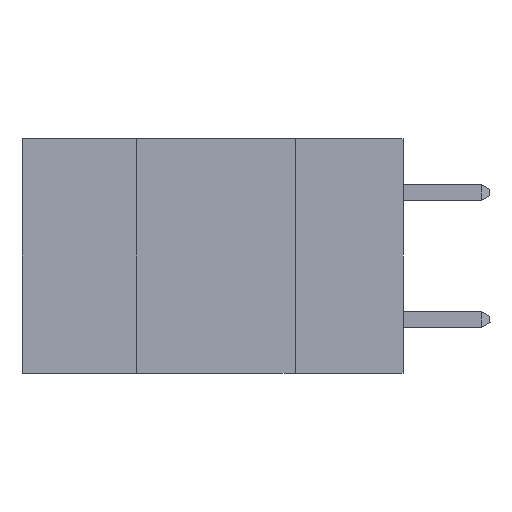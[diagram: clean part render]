
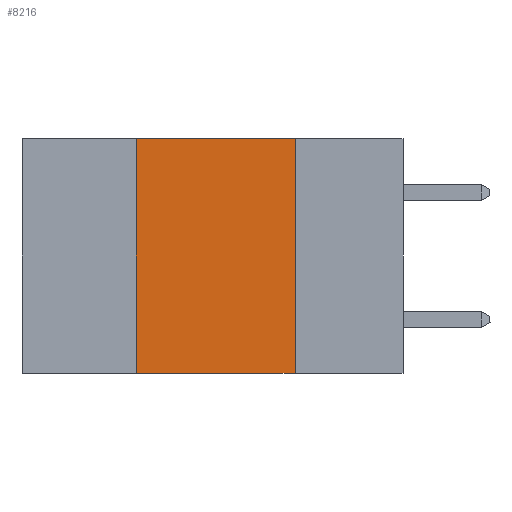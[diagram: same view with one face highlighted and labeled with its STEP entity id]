
A CAD part, left-side view. The second image highlights one B-rep face of the part: STEP entity #8216.
In plain terms, the highlighted planar face has unit normal (-1, 0, 0).
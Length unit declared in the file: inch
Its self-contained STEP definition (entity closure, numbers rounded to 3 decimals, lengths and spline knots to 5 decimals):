
#44 = LINE ( 'NONE', #8003, #1233 ) ;
#308 = DIRECTION ( 'NONE',  ( 0., 0., -1. ) ) ;
#373 = VECTOR ( 'NONE', #1918, 39.37008 ) ;
#449 = CARTESIAN_POINT ( 'NONE',  ( 0., 0.42, 0. ) ) ;
#470 = VERTEX_POINT ( 'NONE', #3989 ) ;
#764 = CARTESIAN_POINT ( 'NONE',  ( 0., 0.6, -0.37 ) ) ;
#1009 = EDGE_CURVE ( 'NONE', #2843, #5276, #44, .T. ) ;
#1233 = VECTOR ( 'NONE', #308, 39.37008 ) ;
#1257 = AXIS2_PLACEMENT_3D ( 'NONE', #8452, #4271, #7788 ) ;
#1403 = CARTESIAN_POINT ( 'NONE',  ( 0., 0.17, -0.37 ) ) ;
#1505 = VECTOR ( 'NONE', #5683, 39.37008 ) ;
#1724 = CARTESIAN_POINT ( 'NONE',  ( 0., 0.6, 0. ) ) ;
#1918 = DIRECTION ( 'NONE',  ( 0., 0., 1. ) ) ;
#1949 = LINE ( 'NONE', #1724, #3927 ) ;
#2248 = LINE ( 'NONE', #449, #373 ) ;
#2525 = VERTEX_POINT ( 'NONE', #7835 ) ;
#2675 = CARTESIAN_POINT ( 'NONE',  ( 0., 0.17, 0. ) ) ;
#2843 = VERTEX_POINT ( 'NONE', #2675 ) ;
#3591 = ORIENTED_EDGE ( 'NONE', *, *, #8362, .T. ) ;
#3927 = VECTOR ( 'NONE', #7334, 39.37008 ) ;
#3989 = CARTESIAN_POINT ( 'NONE',  ( 0., 0.42, -0.37 ) ) ;
#4271 = DIRECTION ( 'NONE',  ( 1., 0., 0. ) ) ;
#4709 = ORIENTED_EDGE ( 'NONE', *, *, #6667, .F. ) ;
#4991 = EDGE_CURVE ( 'NONE', #2525, #2843, #1949, .T. ) ;
#5039 = LINE ( 'NONE', #764, #1505 ) ;
#5276 = VERTEX_POINT ( 'NONE', #1403 ) ;
#5683 = DIRECTION ( 'NONE',  ( 0., -1., 0. ) ) ;
#5774 = ORIENTED_EDGE ( 'NONE', *, *, #1009, .F. ) ;
#6234 = FACE_OUTER_BOUND ( 'NONE', #7098, .T. ) ;
#6667 = EDGE_CURVE ( 'NONE', #470, #2525, #2248, .T. ) ;
#7098 = EDGE_LOOP ( 'NONE', ( #5774, #7159, #4709, #3591 ) ) ;
#7159 = ORIENTED_EDGE ( 'NONE', *, *, #4991, .F. ) ;
#7203 = PLANE ( 'NONE',  #1257 ) ;
#7334 = DIRECTION ( 'NONE',  ( 0., -1., 0. ) ) ;
#7788 = DIRECTION ( 'NONE',  ( 0., 0., -1. ) ) ;
#7835 = CARTESIAN_POINT ( 'NONE',  ( 0., 0.42, 0. ) ) ;
#8003 = CARTESIAN_POINT ( 'NONE',  ( 0., 0.17, 0. ) ) ;
#8216 = ADVANCED_FACE ( 'NONE', ( #6234 ), #7203, .F. ) ;
#8362 = EDGE_CURVE ( 'NONE', #470, #5276, #5039, .T. ) ;
#8452 = CARTESIAN_POINT ( 'NONE',  ( 0., 0.6, 0. ) ) ;
